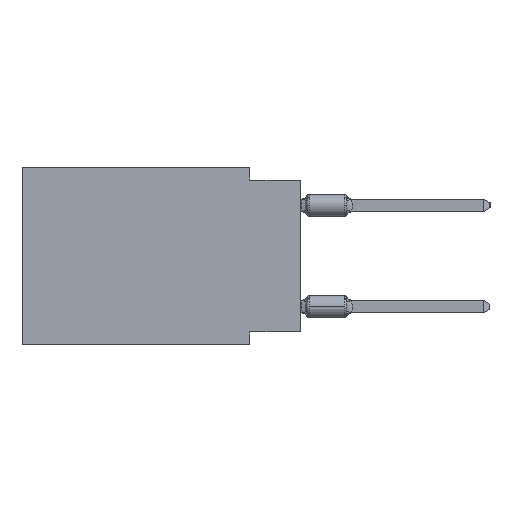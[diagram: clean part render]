
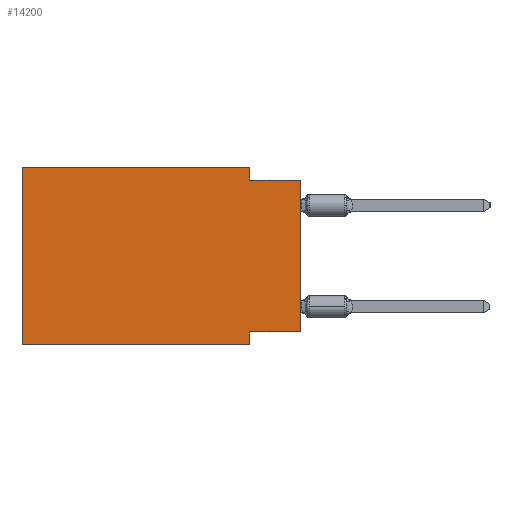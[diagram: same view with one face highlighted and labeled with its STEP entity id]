
A CAD part, left-side view. The second image highlights one B-rep face of the part: STEP entity #14200.
In plain terms, the highlighted planar face has unit normal (-1, 0, 0).
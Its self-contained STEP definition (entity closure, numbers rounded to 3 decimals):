
#124 = DIRECTION ( 'NONE',  ( 0., -1., 0. ) ) ;
#251 = EDGE_CURVE ( 'NONE', #10939, #16749, #11142, .T. ) ;
#299 = CARTESIAN_POINT ( 'NONE',  ( 0., 2.54, -8.255 ) ) ;
#1877 = ORIENTED_EDGE ( 'NONE', *, *, #18208, .F. ) ;
#2010 = VERTEX_POINT ( 'NONE', #15161 ) ;
#2661 = CARTESIAN_POINT ( 'NONE',  ( 0., 2.54, -8.89 ) ) ;
#2693 = EDGE_CURVE ( 'NONE', #14943, #3754, #6887, .T. ) ;
#2885 = CARTESIAN_POINT ( 'NONE',  ( 0., 13.97, 0. ) ) ;
#2927 = LINE ( 'NONE', #2661, #10744 ) ;
#3196 = CARTESIAN_POINT ( 'NONE',  ( 0., 0., -8.255 ) ) ;
#3754 = VERTEX_POINT ( 'NONE', #14226 ) ;
#4107 = CARTESIAN_POINT ( 'NONE',  ( 0., 0., -8.255 ) ) ;
#4180 = EDGE_LOOP ( 'NONE', ( #8447, #14174, #16090, #20889, #19580, #10922, #1877, #6560 ) ) ;
#4298 = VERTEX_POINT ( 'NONE', #17783 ) ;
#4567 = DIRECTION ( 'NONE',  ( 0., 0., 1. ) ) ;
#4625 = DIRECTION ( 'NONE',  ( 0., -1., 0. ) ) ;
#4810 = DIRECTION ( 'NONE',  ( 0., 0., -1. ) ) ;
#4961 = EDGE_CURVE ( 'NONE', #4298, #14943, #5409, .T. ) ;
#5367 = CARTESIAN_POINT ( 'NONE',  ( 0., 0., -0.635 ) ) ;
#5409 = LINE ( 'NONE', #18744, #10449 ) ;
#6246 = DIRECTION ( 'NONE',  ( 1., 0., 0. ) ) ;
#6560 = ORIENTED_EDGE ( 'NONE', *, *, #251, .F. ) ;
#6887 = LINE ( 'NONE', #5367, #10830 ) ;
#8106 = CARTESIAN_POINT ( 'NONE',  ( 0., 13.97, -8.89 ) ) ;
#8137 = PLANE ( 'NONE',  #12731 ) ;
#8149 = CARTESIAN_POINT ( 'NONE',  ( 0., 2.54, -8.89 ) ) ;
#8447 = ORIENTED_EDGE ( 'NONE', *, *, #22910, .T. ) ;
#9064 = EDGE_CURVE ( 'NONE', #2010, #18458, #15449, .T. ) ;
#9115 = CARTESIAN_POINT ( 'NONE',  ( 0., 0., 0. ) ) ;
#9160 = VECTOR ( 'NONE', #16767, 1000. ) ;
#10449 = VECTOR ( 'NONE', #11632, 1000. ) ;
#10562 = VERTEX_POINT ( 'NONE', #2885 ) ;
#10744 = VECTOR ( 'NONE', #4810, 1000. ) ;
#10830 = VECTOR ( 'NONE', #24066, 1000. ) ;
#10922 = ORIENTED_EDGE ( 'NONE', *, *, #9064, .T. ) ;
#10939 = VERTEX_POINT ( 'NONE', #3196 ) ;
#11142 = LINE ( 'NONE', #4107, #9160 ) ;
#11632 = DIRECTION ( 'NONE',  ( 0., 0., -1. ) ) ;
#12729 = DIRECTION ( 'NONE',  ( 0., 0., 1. ) ) ;
#12731 = AXIS2_PLACEMENT_3D ( 'NONE', #22832, #6246, #21435 ) ;
#12772 = VECTOR ( 'NONE', #124, 1000. ) ;
#13550 = EDGE_CURVE ( 'NONE', #2010, #10562, #18039, .T. ) ;
#13854 = FACE_OUTER_BOUND ( 'NONE', #4180, .T. ) ;
#13994 = CARTESIAN_POINT ( 'NONE',  ( 0., 13.97, 0. ) ) ;
#14174 = ORIENTED_EDGE ( 'NONE', *, *, #2693, .F. ) ;
#14200 = ADVANCED_FACE ( 'NONE', ( #13854 ), #8137, .F. ) ;
#14226 = CARTESIAN_POINT ( 'NONE',  ( 0., 0., -0.635 ) ) ;
#14227 = LINE ( 'NONE', #13994, #21879 ) ;
#14354 = EDGE_CURVE ( 'NONE', #10562, #4298, #14227, .T. ) ;
#14355 = LINE ( 'NONE', #9115, #23892 ) ;
#14943 = VERTEX_POINT ( 'NONE', #16456 ) ;
#15161 = CARTESIAN_POINT ( 'NONE',  ( 0., 13.97, -8.89 ) ) ;
#15449 = LINE ( 'NONE', #8106, #12772 ) ;
#16090 = ORIENTED_EDGE ( 'NONE', *, *, #4961, .F. ) ;
#16456 = CARTESIAN_POINT ( 'NONE',  ( 0., 2.54, -0.635 ) ) ;
#16749 = VERTEX_POINT ( 'NONE', #299 ) ;
#16767 = DIRECTION ( 'NONE',  ( 0., 1., 0. ) ) ;
#17783 = CARTESIAN_POINT ( 'NONE',  ( 0., 2.54, 0. ) ) ;
#18039 = LINE ( 'NONE', #23888, #24158 ) ;
#18208 = EDGE_CURVE ( 'NONE', #16749, #18458, #2927, .T. ) ;
#18458 = VERTEX_POINT ( 'NONE', #8149 ) ;
#18744 = CARTESIAN_POINT ( 'NONE',  ( 0., 2.54, 0. ) ) ;
#19580 = ORIENTED_EDGE ( 'NONE', *, *, #13550, .F. ) ;
#20889 = ORIENTED_EDGE ( 'NONE', *, *, #14354, .F. ) ;
#21435 = DIRECTION ( 'NONE',  ( 0., 0., -1. ) ) ;
#21879 = VECTOR ( 'NONE', #4625, 1000. ) ;
#22832 = CARTESIAN_POINT ( 'NONE',  ( 0., 13.97, 0. ) ) ;
#22910 = EDGE_CURVE ( 'NONE', #10939, #3754, #14355, .T. ) ;
#23888 = CARTESIAN_POINT ( 'NONE',  ( 0., 13.97, 0. ) ) ;
#23892 = VECTOR ( 'NONE', #12729, 1000. ) ;
#24066 = DIRECTION ( 'NONE',  ( 0., -1., 0. ) ) ;
#24158 = VECTOR ( 'NONE', #4567, 1000. ) ;
